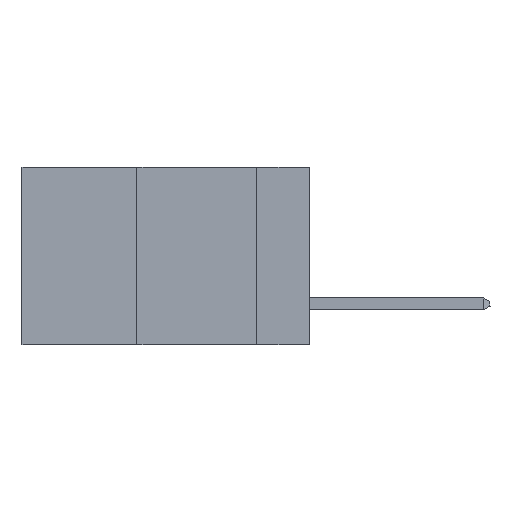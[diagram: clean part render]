
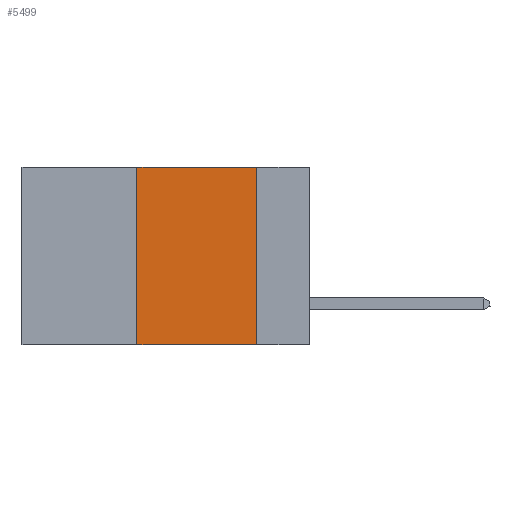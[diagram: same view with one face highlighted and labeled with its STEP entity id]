
A CAD part, left-side view. The second image highlights one B-rep face of the part: STEP entity #5499.
In plain terms, the highlighted planar face has unit normal (-1, 0, 0).
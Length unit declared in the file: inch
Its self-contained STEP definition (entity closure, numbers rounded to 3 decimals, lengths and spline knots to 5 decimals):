
#765 = PLANE ( 'NONE',  #30307 ) ;
#1075 = CARTESIAN_POINT ( 'NONE',  ( 0., 0.11, 0. ) ) ;
#1188 = LINE ( 'NONE', #1075, #21123 ) ;
#1637 = VERTEX_POINT ( 'NONE', #30227 ) ;
#3020 = CARTESIAN_POINT ( 'NONE',  ( 0., 0.6, 0. ) ) ;
#5499 = ADVANCED_FACE ( 'NONE', ( #9330 ), #765, .F. ) ;
#6599 = EDGE_CURVE ( 'NONE', #1637, #12771, #21495, .T. ) ;
#6682 = EDGE_CURVE ( 'NONE', #1637, #23130, #18924, .T. ) ;
#7149 = EDGE_CURVE ( 'NONE', #21170, #12771, #1188, .T. ) ;
#8725 = EDGE_LOOP ( 'NONE', ( #16355, #30494, #19564, #20561 ) ) ;
#9330 = FACE_OUTER_BOUND ( 'NONE', #8725, .T. ) ;
#10092 = VECTOR ( 'NONE', #10494, 39.37008 ) ;
#10275 = DIRECTION ( 'NONE',  ( 1., 0., 0. ) ) ;
#10494 = DIRECTION ( 'NONE',  ( 0., -1., 0. ) ) ;
#10826 = DIRECTION ( 'NONE',  ( 0., 0., 1. ) ) ;
#12664 = DIRECTION ( 'NONE',  ( 0., 0., -1. ) ) ;
#12771 = VERTEX_POINT ( 'NONE', #19722 ) ;
#12963 = LINE ( 'NONE', #30272, #30277 ) ;
#13454 = CARTESIAN_POINT ( 'NONE',  ( 0., 0.36, 0. ) ) ;
#13745 = CARTESIAN_POINT ( 'NONE',  ( 0., 0.11, 0. ) ) ;
#16355 = ORIENTED_EDGE ( 'NONE', *, *, #7149, .F. ) ;
#18924 = LINE ( 'NONE', #13454, #24836 ) ;
#19314 = EDGE_CURVE ( 'NONE', #23130, #21170, #12963, .T. ) ;
#19564 = ORIENTED_EDGE ( 'NONE', *, *, #6682, .F. ) ;
#19722 = CARTESIAN_POINT ( 'NONE',  ( 0., 0.11, -0.37 ) ) ;
#19734 = CARTESIAN_POINT ( 'NONE',  ( 0., 0.36, 0. ) ) ;
#20561 = ORIENTED_EDGE ( 'NONE', *, *, #6599, .T. ) ;
#21123 = VECTOR ( 'NONE', #12664, 39.37008 ) ;
#21170 = VERTEX_POINT ( 'NONE', #13745 ) ;
#21495 = LINE ( 'NONE', #24609, #10092 ) ;
#23130 = VERTEX_POINT ( 'NONE', #19734 ) ;
#24374 = DIRECTION ( 'NONE',  ( 0., 0., -1. ) ) ;
#24609 = CARTESIAN_POINT ( 'NONE',  ( 0., 0.6, -0.37 ) ) ;
#24836 = VECTOR ( 'NONE', #10826, 39.37008 ) ;
#30072 = DIRECTION ( 'NONE',  ( 0., -1., 0. ) ) ;
#30227 = CARTESIAN_POINT ( 'NONE',  ( 0., 0.36, -0.37 ) ) ;
#30272 = CARTESIAN_POINT ( 'NONE',  ( 0., 0.6, 0. ) ) ;
#30277 = VECTOR ( 'NONE', #30072, 39.37008 ) ;
#30307 = AXIS2_PLACEMENT_3D ( 'NONE', #3020, #10275, #24374 ) ;
#30494 = ORIENTED_EDGE ( 'NONE', *, *, #19314, .F. ) ;
